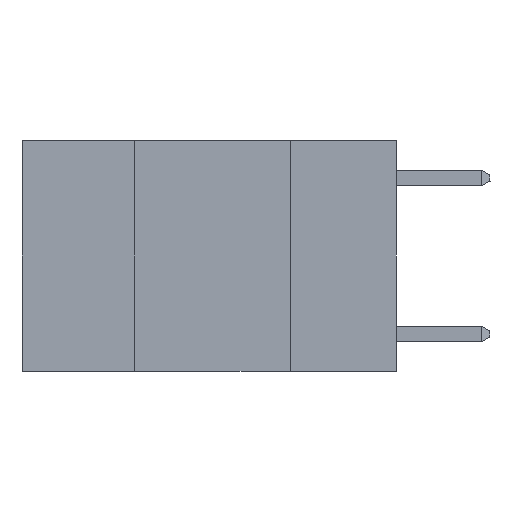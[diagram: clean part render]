
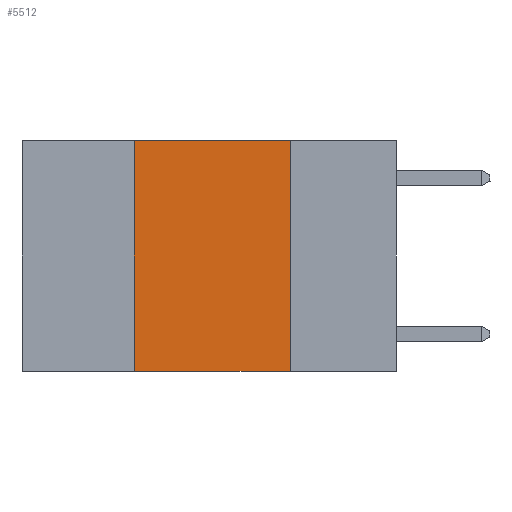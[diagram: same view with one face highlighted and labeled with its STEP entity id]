
A CAD part, left-side view. The second image highlights one B-rep face of the part: STEP entity #5512.
In plain terms, the highlighted planar face has unit normal (-1, 0, 0).
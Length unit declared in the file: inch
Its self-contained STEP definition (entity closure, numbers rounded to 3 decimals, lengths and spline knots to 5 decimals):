
#330 = VERTEX_POINT ( 'NONE', #8261 ) ;
#506 = LINE ( 'NONE', #15415, #5834 ) ;
#1236 = LINE ( 'NONE', #9880, #11883 ) ;
#1407 = DIRECTION ( 'NONE',  ( 0., 0., -1. ) ) ;
#1846 = LINE ( 'NONE', #13548, #6556 ) ;
#2958 = AXIS2_PLACEMENT_3D ( 'NONE', #11961, #5138, #13922 ) ;
#4270 = EDGE_LOOP ( 'NONE', ( #25289, #8056, #18270, #7612 ) ) ;
#4994 = FACE_OUTER_BOUND ( 'NONE', #4270, .T. ) ;
#5138 = DIRECTION ( 'NONE',  ( 1., 0., 0. ) ) ;
#5512 = ADVANCED_FACE ( 'NONE', ( #4994 ), #23623, .F. ) ;
#5834 = VECTOR ( 'NONE', #1407, 39.37008 ) ;
#6556 = VECTOR ( 'NONE', #15532, 39.37008 ) ;
#6693 = LINE ( 'NONE', #24616, #16586 ) ;
#7612 = ORIENTED_EDGE ( 'NONE', *, *, #19603, .T. ) ;
#8056 = ORIENTED_EDGE ( 'NONE', *, *, #16817, .F. ) ;
#8261 = CARTESIAN_POINT ( 'NONE',  ( 0., 0.42, -0.37 ) ) ;
#8973 = DIRECTION ( 'NONE',  ( 0., 0., 1. ) ) ;
#9880 = CARTESIAN_POINT ( 'NONE',  ( 0., 0.6, -0.37 ) ) ;
#11883 = VECTOR ( 'NONE', #23564, 39.37008 ) ;
#11961 = CARTESIAN_POINT ( 'NONE',  ( 0., 0.6, 0. ) ) ;
#11997 = EDGE_CURVE ( 'NONE', #15674, #22024, #506, .T. ) ;
#13548 = CARTESIAN_POINT ( 'NONE',  ( 0., 0.6, 0. ) ) ;
#13922 = DIRECTION ( 'NONE',  ( 0., 0., -1. ) ) ;
#15415 = CARTESIAN_POINT ( 'NONE',  ( 0., 0.17, 0. ) ) ;
#15532 = DIRECTION ( 'NONE',  ( 0., -1., 0. ) ) ;
#15674 = VERTEX_POINT ( 'NONE', #23526 ) ;
#16586 = VECTOR ( 'NONE', #8973, 39.37008 ) ;
#16817 = EDGE_CURVE ( 'NONE', #24702, #15674, #1846, .T. ) ;
#18270 = ORIENTED_EDGE ( 'NONE', *, *, #22956, .F. ) ;
#19603 = EDGE_CURVE ( 'NONE', #330, #22024, #1236, .T. ) ;
#22024 = VERTEX_POINT ( 'NONE', #23229 ) ;
#22956 = EDGE_CURVE ( 'NONE', #330, #24702, #6693, .T. ) ;
#23229 = CARTESIAN_POINT ( 'NONE',  ( 0., 0.17, -0.37 ) ) ;
#23526 = CARTESIAN_POINT ( 'NONE',  ( 0., 0.17, 0. ) ) ;
#23564 = DIRECTION ( 'NONE',  ( 0., -1., 0. ) ) ;
#23623 = PLANE ( 'NONE',  #2958 ) ;
#23868 = CARTESIAN_POINT ( 'NONE',  ( 0., 0.42, 0. ) ) ;
#24616 = CARTESIAN_POINT ( 'NONE',  ( 0., 0.42, 0. ) ) ;
#24702 = VERTEX_POINT ( 'NONE', #23868 ) ;
#25289 = ORIENTED_EDGE ( 'NONE', *, *, #11997, .F. ) ;
